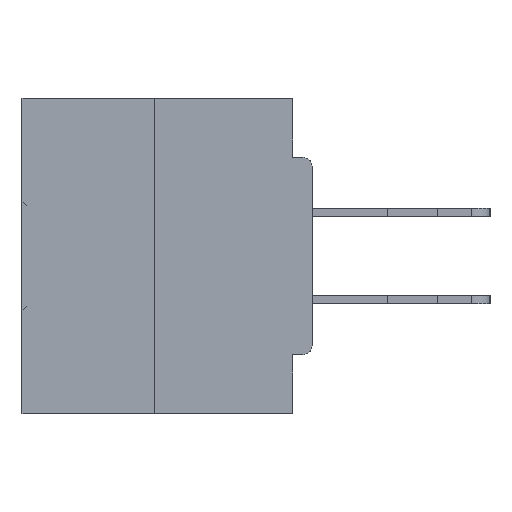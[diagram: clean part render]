
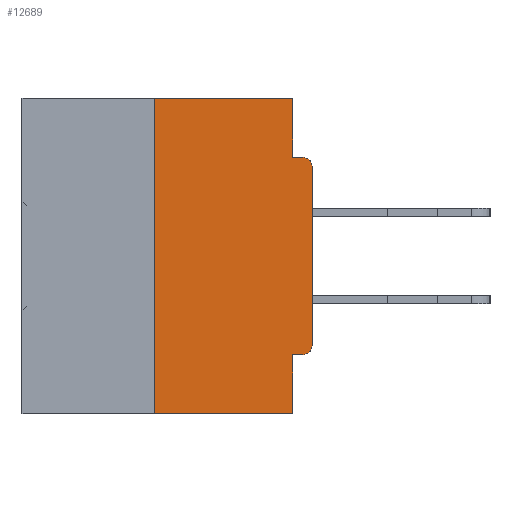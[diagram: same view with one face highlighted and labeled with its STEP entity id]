
A CAD part, left-side view. The second image highlights one B-rep face of the part: STEP entity #12689.
In plain terms, the highlighted planar face has unit normal (-1, 0, 0).
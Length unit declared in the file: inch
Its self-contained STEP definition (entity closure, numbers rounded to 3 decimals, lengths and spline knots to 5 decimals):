
#723 = LINE ( 'NONE', #44164, #10024 ) ;
#1030 = CIRCLE ( 'NONE', #2552, 0.015 ) ;
#2463 = ORIENTED_EDGE ( 'NONE', *, *, #34758, .F. ) ;
#2552 = AXIS2_PLACEMENT_3D ( 'NONE', #35648, #17617, #24956 ) ;
#3294 = AXIS2_PLACEMENT_3D ( 'NONE', #26717, #36922, #4428 ) ;
#4428 = DIRECTION ( 'NONE',  ( 0., 0., -1. ) ) ;
#5220 = EDGE_CURVE ( 'NONE', #18474, #37291, #6749, .T. ) ;
#5391 = DIRECTION ( 'NONE',  ( 0., 0., 1. ) ) ;
#5814 = EDGE_CURVE ( 'NONE', #32262, #46812, #723, .T. ) ;
#5896 = FACE_OUTER_BOUND ( 'NONE', #23499, .T. ) ;
#6177 = EDGE_CURVE ( 'NONE', #22056, #18474, #36494, .T. ) ;
#6749 = LINE ( 'NONE', #21193, #22806 ) ;
#7749 = CARTESIAN_POINT ( 'NONE',  ( 0., 0., -0.3915 ) ) ;
#8396 = CARTESIAN_POINT ( 'NONE',  ( 0., 0., -0.0935 ) ) ;
#8658 = DIRECTION ( 'NONE',  ( 0., 0., 1. ) ) ;
#10024 = VECTOR ( 'NONE', #44388, 39.37008 ) ;
#10118 = CARTESIAN_POINT ( 'NONE',  ( 0., 0.015, -0.4065 ) ) ;
#11052 = DIRECTION ( 'NONE',  ( 0., 0., -1. ) ) ;
#11387 = DIRECTION ( 'NONE',  ( 0., -1., 0. ) ) ;
#12264 = EDGE_CURVE ( 'NONE', #42086, #22056, #19779, .T. ) ;
#12689 = ADVANCED_FACE ( 'NONE', ( #5896 ), #16555, .F. ) ;
#13831 = VECTOR ( 'NONE', #11387, 39.37008 ) ;
#14161 = VECTOR ( 'NONE', #8658, 39.37008 ) ;
#15055 = DIRECTION ( 'NONE',  ( 0., -1., 0. ) ) ;
#15133 = CARTESIAN_POINT ( 'NONE',  ( 0., 0.015, -0.0935 ) ) ;
#15271 = LINE ( 'NONE', #8396, #24967 ) ;
#15462 = DIRECTION ( 'NONE',  ( 1., 0., 0. ) ) ;
#16181 = CIRCLE ( 'NONE', #3294, 0.015 ) ;
#16278 = LINE ( 'NONE', #38331, #28245 ) ;
#16442 = CARTESIAN_POINT ( 'NONE',  ( 0., 0.25, 0. ) ) ;
#16555 = PLANE ( 'NONE',  #46033 ) ;
#16862 = ORIENTED_EDGE ( 'NONE', *, *, #27734, .T. ) ;
#17617 = DIRECTION ( 'NONE',  ( -1., 0., 0. ) ) ;
#17953 = EDGE_CURVE ( 'NONE', #37291, #35706, #15271, .T. ) ;
#17986 = ORIENTED_EDGE ( 'NONE', *, *, #5814, .F. ) ;
#18474 = VERTEX_POINT ( 'NONE', #32731 ) ;
#18569 = DIRECTION ( 'NONE',  ( 0., -1., 0. ) ) ;
#19329 = VERTEX_POINT ( 'NONE', #7749 ) ;
#19779 = LINE ( 'NONE', #16442, #14161 ) ;
#20894 = CARTESIAN_POINT ( 'NONE',  ( 0., 0., -0.1085 ) ) ;
#21193 = CARTESIAN_POINT ( 'NONE',  ( 0., 0.031, 0. ) ) ;
#22056 = VERTEX_POINT ( 'NONE', #35230 ) ;
#22763 = VERTEX_POINT ( 'NONE', #37282 ) ;
#22806 = VECTOR ( 'NONE', #31639, 39.37008 ) ;
#23497 = VECTOR ( 'NONE', #15055, 39.37008 ) ;
#23499 = EDGE_LOOP ( 'NONE', ( #32045, #41284, #25024, #2463, #17986, #16862, #30742, #33177, #24832, #40740 ) ) ;
#24832 = ORIENTED_EDGE ( 'NONE', *, *, #17953, .F. ) ;
#24956 = DIRECTION ( 'NONE',  ( 0., 0., -1. ) ) ;
#24967 = VECTOR ( 'NONE', #18569, 39.37008 ) ;
#25024 = ORIENTED_EDGE ( 'NONE', *, *, #38160, .T. ) ;
#25946 = CARTESIAN_POINT ( 'NONE',  ( 0., 0.46, -0.5 ) ) ;
#26413 = CARTESIAN_POINT ( 'NONE',  ( 0., 0.031, -0.5 ) ) ;
#26717 = CARTESIAN_POINT ( 'NONE',  ( 0., 0.015, -0.3915 ) ) ;
#27734 = EDGE_CURVE ( 'NONE', #32262, #19329, #16181, .T. ) ;
#27915 = CARTESIAN_POINT ( 'NONE',  ( 0., 0.46, 0. ) ) ;
#28245 = VECTOR ( 'NONE', #5391, 39.37008 ) ;
#30742 = ORIENTED_EDGE ( 'NONE', *, *, #39195, .T. ) ;
#31639 = DIRECTION ( 'NONE',  ( 0., 0., -1. ) ) ;
#32045 = ORIENTED_EDGE ( 'NONE', *, *, #6177, .F. ) ;
#32262 = VERTEX_POINT ( 'NONE', #10118 ) ;
#32731 = CARTESIAN_POINT ( 'NONE',  ( 0., 0.031, 0. ) ) ;
#32913 = CARTESIAN_POINT ( 'NONE',  ( 0., 0.46, 0. ) ) ;
#33177 = ORIENTED_EDGE ( 'NONE', *, *, #39923, .T. ) ;
#33295 = LINE ( 'NONE', #25946, #23497 ) ;
#34758 = EDGE_CURVE ( 'NONE', #46812, #22763, #40915, .T. ) ;
#35230 = CARTESIAN_POINT ( 'NONE',  ( 0., 0.25, 0. ) ) ;
#35477 = VECTOR ( 'NONE', #11052, 39.37008 ) ;
#35648 = CARTESIAN_POINT ( 'NONE',  ( 0., 0.015, -0.1085 ) ) ;
#35706 = VERTEX_POINT ( 'NONE', #15133 ) ;
#36115 = CARTESIAN_POINT ( 'NONE',  ( 0., 0.25, -0.5 ) ) ;
#36494 = LINE ( 'NONE', #32913, #13831 ) ;
#36922 = DIRECTION ( 'NONE',  ( -1., 0., 0. ) ) ;
#37282 = CARTESIAN_POINT ( 'NONE',  ( 0., 0.031, -0.5 ) ) ;
#37291 = VERTEX_POINT ( 'NONE', #46184 ) ;
#38160 = EDGE_CURVE ( 'NONE', #42086, #22763, #33295, .T. ) ;
#38331 = CARTESIAN_POINT ( 'NONE',  ( 0., 0., 0. ) ) ;
#39195 = EDGE_CURVE ( 'NONE', #19329, #43605, #16278, .T. ) ;
#39923 = EDGE_CURVE ( 'NONE', #43605, #35706, #1030, .T. ) ;
#40249 = CARTESIAN_POINT ( 'NONE',  ( 0., 0.031, -0.4065 ) ) ;
#40740 = ORIENTED_EDGE ( 'NONE', *, *, #5220, .F. ) ;
#40915 = LINE ( 'NONE', #26413, #35477 ) ;
#41284 = ORIENTED_EDGE ( 'NONE', *, *, #12264, .F. ) ;
#42086 = VERTEX_POINT ( 'NONE', #36115 ) ;
#43605 = VERTEX_POINT ( 'NONE', #20894 ) ;
#44164 = CARTESIAN_POINT ( 'NONE',  ( 0., 0., -0.4065 ) ) ;
#44388 = DIRECTION ( 'NONE',  ( 0., 1., 0. ) ) ;
#45976 = DIRECTION ( 'NONE',  ( 0., 0., -1. ) ) ;
#46033 = AXIS2_PLACEMENT_3D ( 'NONE', #27915, #15462, #45976 ) ;
#46184 = CARTESIAN_POINT ( 'NONE',  ( 0., 0.031, -0.0935 ) ) ;
#46812 = VERTEX_POINT ( 'NONE', #40249 ) ;
